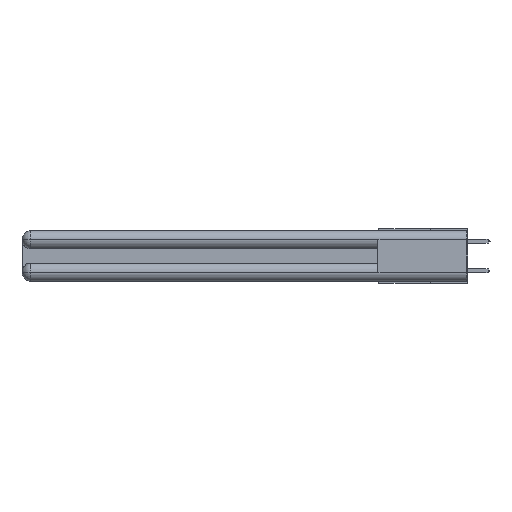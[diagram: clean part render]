
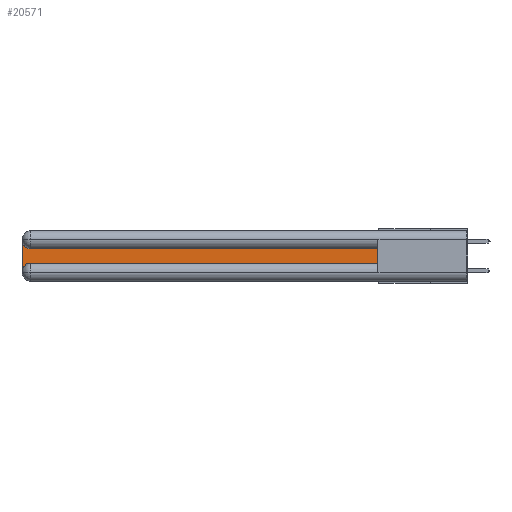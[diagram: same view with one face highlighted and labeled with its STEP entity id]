
A CAD part, left-side view. The second image highlights one B-rep face of the part: STEP entity #20571.
In plain terms, the highlighted planar face has unit normal (-1, 0, 0).
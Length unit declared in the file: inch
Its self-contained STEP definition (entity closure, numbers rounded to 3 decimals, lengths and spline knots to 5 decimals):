
#617 = VERTEX_POINT ( 'NONE', #3260 ) ;
#646 = AXIS2_PLACEMENT_3D ( 'NONE', #9258, #24836, #15950 ) ;
#2169 = LINE ( 'NONE', #18246, #3946 ) ;
#2217 = CARTESIAN_POINT ( 'NONE',  ( 0.075, 2.94, -0.1225 ) ) ;
#3260 = CARTESIAN_POINT ( 'NONE',  ( 0.075, 2.94, -0.2175 ) ) ;
#3657 = CARTESIAN_POINT ( 'NONE',  ( 0.075, 3., -0.2775 ) ) ;
#3797 = EDGE_CURVE ( 'NONE', #617, #14432, #19143, .T. ) ;
#3946 = VECTOR ( 'NONE', #22703, 39.37008 ) ;
#3969 = CARTESIAN_POINT ( 'NONE',  ( 0.075, 0.6, -0.1225 ) ) ;
#4312 = VERTEX_POINT ( 'NONE', #8120 ) ;
#4350 = CARTESIAN_POINT ( 'NONE',  ( 0.075, 3., -0.1225 ) ) ;
#4597 = VERTEX_POINT ( 'NONE', #2217 ) ;
#5494 = ORIENTED_EDGE ( 'NONE', *, *, #23493, .T. ) ;
#5588 = CARTESIAN_POINT ( 'NONE',  ( 0.075, 3., -0.2175 ) ) ;
#6999 = ORIENTED_EDGE ( 'NONE', *, *, #19448, .T. ) ;
#8120 = CARTESIAN_POINT ( 'NONE',  ( 0.075, 3., -0.0625 ) ) ;
#8488 = DIRECTION ( 'NONE',  ( 1., 0., 0. ) ) ;
#8877 = DIRECTION ( 'NONE',  ( 0., 0., -1. ) ) ;
#9253 = EDGE_CURVE ( 'NONE', #14432, #26601, #18528, .T. ) ;
#9258 = CARTESIAN_POINT ( 'NONE',  ( 0.075, 2.94, -0.2775 ) ) ;
#11068 = DIRECTION ( 'NONE',  ( 0., 0., -1. ) ) ;
#11717 = ORIENTED_EDGE ( 'NONE', *, *, #3797, .T. ) ;
#12194 = CARTESIAN_POINT ( 'NONE',  ( 0.075, 0.6, -0.2175 ) ) ;
#12314 = CIRCLE ( 'NONE', #646, 0.06 ) ;
#12417 = EDGE_LOOP ( 'NONE', ( #22105, #6999, #27726, #5494, #11717, #19017 ) ) ;
#12516 = VECTOR ( 'NONE', #26328, 39.37008 ) ;
#12655 = AXIS2_PLACEMENT_3D ( 'NONE', #4350, #8488, #11068 ) ;
#14432 = VERTEX_POINT ( 'NONE', #12194 ) ;
#14901 = LINE ( 'NONE', #5588, #25000 ) ;
#14908 = DIRECTION ( 'NONE',  ( 0., 0., -1. ) ) ;
#15950 = DIRECTION ( 'NONE',  ( 0., 0., -1. ) ) ;
#16079 = EDGE_CURVE ( 'NONE', #4312, #18823, #14901, .T. ) ;
#17105 = EDGE_CURVE ( 'NONE', #26601, #4597, #2169, .T. ) ;
#17131 = CARTESIAN_POINT ( 'NONE',  ( 0.075, 0.6, -0.2175 ) ) ;
#17469 = AXIS2_PLACEMENT_3D ( 'NONE', #22102, #24337, #8877 ) ;
#18246 = CARTESIAN_POINT ( 'NONE',  ( 0.075, 0.6, -0.1225 ) ) ;
#18528 = LINE ( 'NONE', #17131, #19927 ) ;
#18823 = VERTEX_POINT ( 'NONE', #3657 ) ;
#19017 = ORIENTED_EDGE ( 'NONE', *, *, #9253, .T. ) ;
#19143 = LINE ( 'NONE', #21841, #12516 ) ;
#19246 = FACE_OUTER_BOUND ( 'NONE', #12417, .T. ) ;
#19448 = EDGE_CURVE ( 'NONE', #4597, #4312, #27377, .T. ) ;
#19927 = VECTOR ( 'NONE', #28061, 39.37008 ) ;
#20571 = ADVANCED_FACE ( 'NONE', ( #19246 ), #24328, .F. ) ;
#21841 = CARTESIAN_POINT ( 'NONE',  ( 0.075, 0.6, -0.2175 ) ) ;
#22102 = CARTESIAN_POINT ( 'NONE',  ( 0.075, 2.94, -0.0625 ) ) ;
#22105 = ORIENTED_EDGE ( 'NONE', *, *, #17105, .T. ) ;
#22703 = DIRECTION ( 'NONE',  ( 0., 1., 0. ) ) ;
#23493 = EDGE_CURVE ( 'NONE', #18823, #617, #12314, .T. ) ;
#24328 = PLANE ( 'NONE',  #12655 ) ;
#24337 = DIRECTION ( 'NONE',  ( 1., 0., 0. ) ) ;
#24836 = DIRECTION ( 'NONE',  ( 1., 0., 0. ) ) ;
#25000 = VECTOR ( 'NONE', #14908, 39.37008 ) ;
#26328 = DIRECTION ( 'NONE',  ( 0., -1., 0. ) ) ;
#26601 = VERTEX_POINT ( 'NONE', #3969 ) ;
#27377 = CIRCLE ( 'NONE', #17469, 0.06 ) ;
#27726 = ORIENTED_EDGE ( 'NONE', *, *, #16079, .T. ) ;
#28061 = DIRECTION ( 'NONE',  ( 0., 0., 1. ) ) ;
